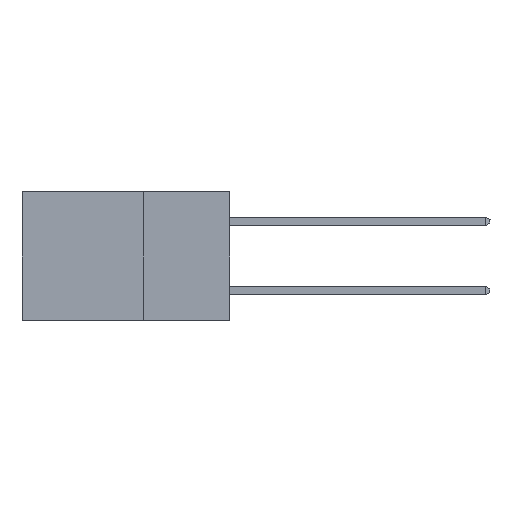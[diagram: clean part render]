
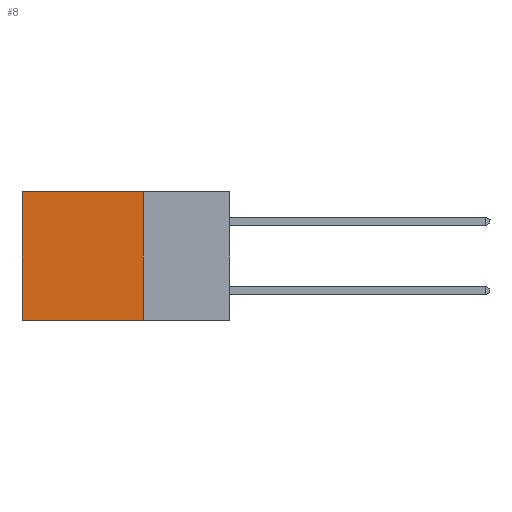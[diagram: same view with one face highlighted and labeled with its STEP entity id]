
A CAD part, left-side view. The second image highlights one B-rep face of the part: STEP entity #8.
In plain terms, the highlighted planar face has unit normal (-1, 0, 0).
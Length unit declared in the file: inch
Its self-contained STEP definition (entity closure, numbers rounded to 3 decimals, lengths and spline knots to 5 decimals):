
#8 = ADVANCED_FACE ( 'NONE', ( #723 ), #9267, .F. ) ;
#266 = CARTESIAN_POINT ( 'NONE',  ( 0.2615, 0.6, 0. ) ) ;
#723 = FACE_OUTER_BOUND ( 'NONE', #8086, .T. ) ;
#988 = VECTOR ( 'NONE', #10193, 39.37008 ) ;
#1131 = LINE ( 'NONE', #2357, #988 ) ;
#2195 = EDGE_CURVE ( 'NONE', #10251, #3903, #4203, .T. ) ;
#2318 = CARTESIAN_POINT ( 'NONE',  ( 0.2615, 0.25, -0.37 ) ) ;
#2357 = CARTESIAN_POINT ( 'NONE',  ( 0.2615, 0.25, -0.37 ) ) ;
#2650 = VECTOR ( 'NONE', #3966, 39.37008 ) ;
#2781 = DIRECTION ( 'NONE',  ( 0., 0., -1. ) ) ;
#3627 = ORIENTED_EDGE ( 'NONE', *, *, #2195, .T. ) ;
#3903 = VERTEX_POINT ( 'NONE', #266 ) ;
#3966 = DIRECTION ( 'NONE',  ( 0., 1., 0. ) ) ;
#4203 = LINE ( 'NONE', #8249, #12569 ) ;
#4423 = CARTESIAN_POINT ( 'NONE',  ( 0.2615, 0.6, -0.37 ) ) ;
#4650 = LINE ( 'NONE', #4715, #11825 ) ;
#4652 = CARTESIAN_POINT ( 'NONE',  ( 0.2615, 0.25, 0. ) ) ;
#4715 = CARTESIAN_POINT ( 'NONE',  ( 0.2615, 0.6, -0.37 ) ) ;
#4944 = LINE ( 'NONE', #6670, #2650 ) ;
#6670 = CARTESIAN_POINT ( 'NONE',  ( 0.2615, 0.25, -0.37 ) ) ;
#7325 = EDGE_CURVE ( 'NONE', #3903, #12492, #4650, .T. ) ;
#7637 = ORIENTED_EDGE ( 'NONE', *, *, #8394, .F. ) ;
#8060 = EDGE_CURVE ( 'NONE', #10251, #12041, #1131, .T. ) ;
#8086 = EDGE_LOOP ( 'NONE', ( #10454, #7637, #9675, #3627 ) ) ;
#8249 = CARTESIAN_POINT ( 'NONE',  ( 0.2615, 0.25, 0. ) ) ;
#8394 = EDGE_CURVE ( 'NONE', #12041, #12492, #4944, .T. ) ;
#8446 = DIRECTION ( 'NONE',  ( 1., 0., 0. ) ) ;
#9267 = PLANE ( 'NONE',  #12531 ) ;
#9392 = DIRECTION ( 'NONE',  ( 0., 0., -1. ) ) ;
#9675 = ORIENTED_EDGE ( 'NONE', *, *, #8060, .F. ) ;
#10193 = DIRECTION ( 'NONE',  ( 0., 0., -1. ) ) ;
#10235 = CARTESIAN_POINT ( 'NONE',  ( 0.2615, 0.25, -0.37 ) ) ;
#10251 = VERTEX_POINT ( 'NONE', #4652 ) ;
#10454 = ORIENTED_EDGE ( 'NONE', *, *, #7325, .T. ) ;
#10993 = DIRECTION ( 'NONE',  ( 0., 1., 0. ) ) ;
#11825 = VECTOR ( 'NONE', #2781, 39.37008 ) ;
#12041 = VERTEX_POINT ( 'NONE', #2318 ) ;
#12492 = VERTEX_POINT ( 'NONE', #4423 ) ;
#12531 = AXIS2_PLACEMENT_3D ( 'NONE', #10235, #8446, #9392 ) ;
#12569 = VECTOR ( 'NONE', #10993, 39.37008 ) ;
